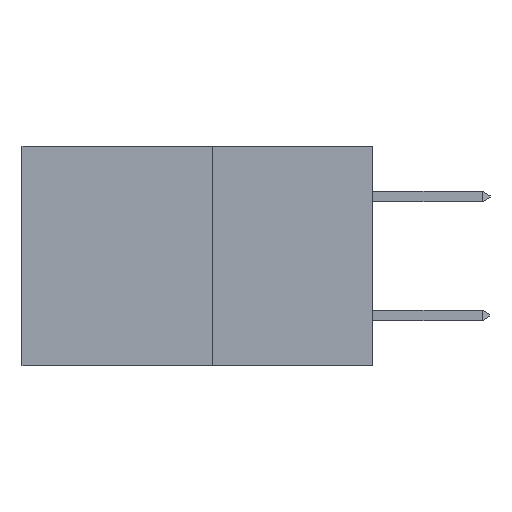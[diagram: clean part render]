
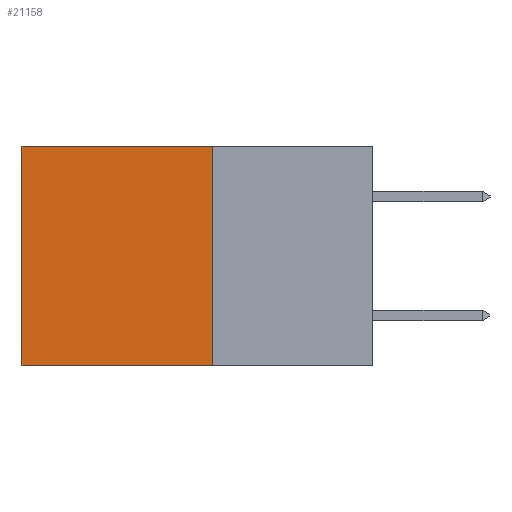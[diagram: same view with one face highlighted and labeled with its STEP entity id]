
A CAD part, left-side view. The second image highlights one B-rep face of the part: STEP entity #21158.
In plain terms, the highlighted planar face has unit normal (-1, 0, 0).
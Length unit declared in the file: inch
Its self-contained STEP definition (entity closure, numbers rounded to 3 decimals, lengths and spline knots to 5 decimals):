
#731 = CARTESIAN_POINT ( 'NONE',  ( 0.277, 0.59, -0.37 ) ) ;
#840 = PLANE ( 'NONE',  #18711 ) ;
#1020 = VERTEX_POINT ( 'NONE', #1814 ) ;
#1250 = EDGE_CURVE ( 'NONE', #1020, #9367, #7953, .T. ) ;
#1814 = CARTESIAN_POINT ( 'NONE',  ( 0.277, 0.27, 0. ) ) ;
#1930 = LINE ( 'NONE', #20933, #10729 ) ;
#2668 = DIRECTION ( 'NONE',  ( 1., 0., 0. ) ) ;
#2866 = VERTEX_POINT ( 'NONE', #9120 ) ;
#3034 = ORIENTED_EDGE ( 'NONE', *, *, #1250, .F. ) ;
#3381 = LINE ( 'NONE', #19582, #17376 ) ;
#3478 = ORIENTED_EDGE ( 'NONE', *, *, #4836, .T. ) ;
#3936 = DIRECTION ( 'NONE',  ( 0., 1., 0. ) ) ;
#4120 = EDGE_LOOP ( 'NONE', ( #15745, #21776, #3034, #3478 ) ) ;
#4394 = CARTESIAN_POINT ( 'NONE',  ( 0.277, 0.27, -0.37 ) ) ;
#4836 = EDGE_CURVE ( 'NONE', #1020, #2866, #1930, .T. ) ;
#6859 = LINE ( 'NONE', #731, #10924 ) ;
#6975 = EDGE_CURVE ( 'NONE', #2866, #14354, #6859, .T. ) ;
#7637 = FACE_OUTER_BOUND ( 'NONE', #4120, .T. ) ;
#7953 = LINE ( 'NONE', #11803, #12111 ) ;
#8787 = CARTESIAN_POINT ( 'NONE',  ( 0.277, 0.59, -0.37 ) ) ;
#9120 = CARTESIAN_POINT ( 'NONE',  ( 0.277, 0.59, 0. ) ) ;
#9367 = VERTEX_POINT ( 'NONE', #10582 ) ;
#10582 = CARTESIAN_POINT ( 'NONE',  ( 0.277, 0.27, -0.37 ) ) ;
#10729 = VECTOR ( 'NONE', #15257, 39.37008 ) ;
#10924 = VECTOR ( 'NONE', #13233, 39.37008 ) ;
#11803 = CARTESIAN_POINT ( 'NONE',  ( 0.277, 0.27, -0.37 ) ) ;
#12111 = VECTOR ( 'NONE', #15953, 39.37008 ) ;
#13233 = DIRECTION ( 'NONE',  ( 0., 0., -1. ) ) ;
#14354 = VERTEX_POINT ( 'NONE', #8787 ) ;
#14492 = EDGE_CURVE ( 'NONE', #9367, #14354, #3381, .T. ) ;
#15008 = DIRECTION ( 'NONE',  ( 0., 0., -1. ) ) ;
#15257 = DIRECTION ( 'NONE',  ( 0., 1., 0. ) ) ;
#15745 = ORIENTED_EDGE ( 'NONE', *, *, #6975, .T. ) ;
#15953 = DIRECTION ( 'NONE',  ( 0., 0., -1. ) ) ;
#17376 = VECTOR ( 'NONE', #3936, 39.37008 ) ;
#18711 = AXIS2_PLACEMENT_3D ( 'NONE', #4394, #2668, #15008 ) ;
#19582 = CARTESIAN_POINT ( 'NONE',  ( 0.277, 0.27, -0.37 ) ) ;
#20933 = CARTESIAN_POINT ( 'NONE',  ( 0.277, 0.27, 0. ) ) ;
#21158 = ADVANCED_FACE ( 'NONE', ( #7637 ), #840, .F. ) ;
#21776 = ORIENTED_EDGE ( 'NONE', *, *, #14492, .F. ) ;
